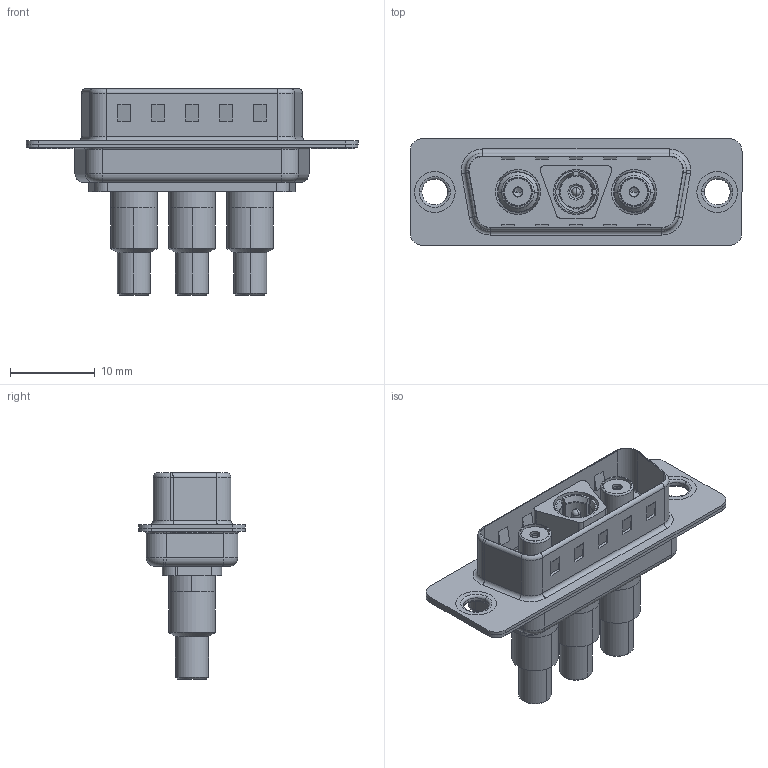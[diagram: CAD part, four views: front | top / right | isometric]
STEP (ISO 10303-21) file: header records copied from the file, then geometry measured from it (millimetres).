
FILE_DESCRIPTION (( 'STEP AP203' ), '1' );
FILE_NAME ('627-3WK3622-5N1.STEP', '2019-05-24T23:15:40', ( '' ), ( '' ), 'SwSTEP 2.0', 'SolidWorks 2016', '' );
FILE_SCHEMA (( 'CONFIG_CONTROL_DESIGN' ));
Length unit declared in the file: millimetre
Products named in the file (16): Insulator Socket; 627Combo Thru Hole Rivet; Insulator Socket 2; Co-Ax Plug_Solder Cup Tail; Socket_Solder Cup; Insulator Pin_Solder Cup Tail; Co-Ax Jack Assy_SC; Pin_Solder Cup; 627-3WK3622-5N1; Locking Collar; Solder Cover; 627Combo Housing_3WK3; Co-Ax Plug Assy_SC; 627Combo Shell Rear_15 Contacts; Co-Ax Jack_Solder Cup Tail; 627Combo Shell Front_15 Contacts
Assembly tree (19 placements, depth 3):
  627-3WK3622-5N1
    627Combo Housing_3WK3
    627Combo Shell Rear_15 Contacts
    627Combo Shell Front_15 Contacts
    627Combo Thru Hole Rivet  x2
    Co-Ax Plug Assy_SC
      Co-Ax Plug_Solder Cup Tail
      Insulator Pin_Solder Cup Tail
      Pin_Solder Cup
      Locking Collar
      Solder Cover
    Co-Ax Jack Assy_SC  x2
      Co-Ax Jack_Solder Cup Tail
      Insulator Socket
      Insulator Socket 2
      Locking Collar
      Socket_Solder Cup
      Solder Cover
Bounding box: 39.15 x 12.6 x 24.3 mm (x, y, z)
Volume: 2264.9 mm3; surface area: 7249.3 mm2
Topology: 22 solids, 22 shells, 730 faces, 1725 edges, 1066 vertices
Faces by surface type: cylinder 312, plane 274, torus 70, cone 66, bspline 6, sphere 2
Entity records: 18466 total; most frequent: CARTESIAN_POINT 3089, DIRECTION 3051, ORIENTED_EDGE 2686, EDGE_CURVE 1343, AXIS2_PLACEMENT_3D 1173, VERTEX_POINT 842, LINE 705, VECTOR 705
